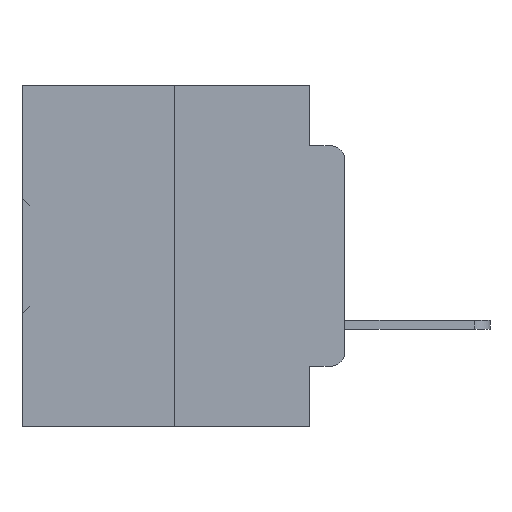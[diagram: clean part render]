
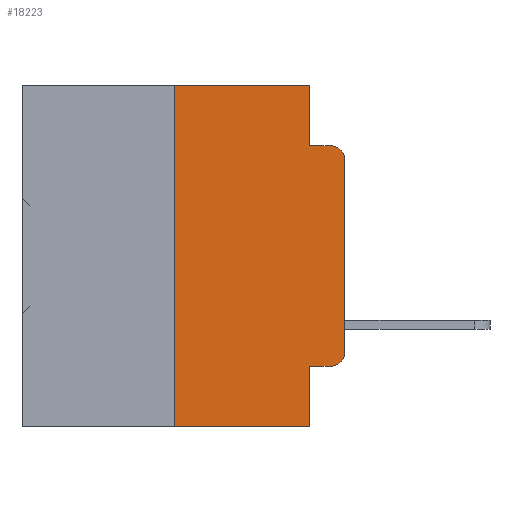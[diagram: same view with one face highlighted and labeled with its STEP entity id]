
A CAD part, left-side view. The second image highlights one B-rep face of the part: STEP entity #18223.
In plain terms, the highlighted planar face has unit normal (-1, 0, 0).
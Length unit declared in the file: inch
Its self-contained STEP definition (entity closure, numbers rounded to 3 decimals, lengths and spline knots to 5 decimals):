
#639 = VERTEX_POINT ( 'NONE', #9170 ) ;
#1669 = VECTOR ( 'NONE', #2910, 39.37008 ) ;
#1952 = CARTESIAN_POINT ( 'NONE',  ( 0., 0.25, 0. ) ) ;
#2910 = DIRECTION ( 'NONE',  ( 0., -1., 0. ) ) ;
#3035 = CARTESIAN_POINT ( 'NONE',  ( 0., 0.473, 0. ) ) ;
#3093 = DIRECTION ( 'NONE',  ( 0., 0., -1. ) ) ;
#4066 = CARTESIAN_POINT ( 'NONE',  ( 0., 0.02, -0.3915 ) ) ;
#5423 = DIRECTION ( 'NONE',  ( 0., -1., 0. ) ) ;
#5424 = VECTOR ( 'NONE', #35236, 39.37008 ) ;
#6036 = LINE ( 'NONE', #36632, #36297 ) ;
#6389 = DIRECTION ( 'NONE',  ( 1., 0., 0. ) ) ;
#6413 = EDGE_CURVE ( 'NONE', #38386, #11973, #16424, .T. ) ;
#7213 = VECTOR ( 'NONE', #23449, 39.37008 ) ;
#7255 = DIRECTION ( 'NONE',  ( 0., 0., -1. ) ) ;
#7344 = LINE ( 'NONE', #27933, #22648 ) ;
#7546 = DIRECTION ( 'NONE',  ( 0., -1., 0. ) ) ;
#7761 = VECTOR ( 'NONE', #5423, 39.37008 ) ;
#7992 = AXIS2_PLACEMENT_3D ( 'NONE', #4066, #25380, #7255 ) ;
#8568 = ORIENTED_EDGE ( 'NONE', *, *, #12694, .F. ) ;
#8886 = EDGE_LOOP ( 'NONE', ( #9324, #9096, #8568, #9856, #9718, #10100, #32846, #32036, #26861, #32527 ) ) ;
#9096 = ORIENTED_EDGE ( 'NONE', *, *, #18917, .T. ) ;
#9102 = VECTOR ( 'NONE', #36524, 39.37008 ) ;
#9170 = CARTESIAN_POINT ( 'NONE',  ( 0., 0.051, 0. ) ) ;
#9175 = VERTEX_POINT ( 'NONE', #12845 ) ;
#9254 = EDGE_CURVE ( 'NONE', #23897, #35153, #20009, .T. ) ;
#9324 = ORIENTED_EDGE ( 'NONE', *, *, #22839, .T. ) ;
#9718 = ORIENTED_EDGE ( 'NONE', *, *, #37402, .F. ) ;
#9856 = ORIENTED_EDGE ( 'NONE', *, *, #10630, .F. ) ;
#10017 = DIRECTION ( 'NONE',  ( -1., 0., 0. ) ) ;
#10100 = ORIENTED_EDGE ( 'NONE', *, *, #6413, .F. ) ;
#10434 = AXIS2_PLACEMENT_3D ( 'NONE', #3035, #6389, #27438 ) ;
#10630 = EDGE_CURVE ( 'NONE', #639, #30252, #28795, .T. ) ;
#11113 = LINE ( 'NONE', #24247, #1669 ) ;
#11973 = VERTEX_POINT ( 'NONE', #1952 ) ;
#12105 = CARTESIAN_POINT ( 'NONE',  ( 0., 0.473, -0.5 ) ) ;
#12694 = EDGE_CURVE ( 'NONE', #30252, #18925, #11113, .T. ) ;
#12845 = CARTESIAN_POINT ( 'NONE',  ( 0., 0.051, -0.5 ) ) ;
#14401 = CARTESIAN_POINT ( 'NONE',  ( 0., 0.25, 0. ) ) ;
#14724 = LINE ( 'NONE', #12105, #5424 ) ;
#14853 = CARTESIAN_POINT ( 'NONE',  ( 0., 0.473, 0. ) ) ;
#15561 = VERTEX_POINT ( 'NONE', #34172 ) ;
#15865 = CARTESIAN_POINT ( 'NONE',  ( 0., 0., -0.3915 ) ) ;
#16025 = LINE ( 'NONE', #14853, #7761 ) ;
#16424 = LINE ( 'NONE', #14401, #7213 ) ;
#18223 = ADVANCED_FACE ( 'NONE', ( #33778 ), #38359, .F. ) ;
#18917 = EDGE_CURVE ( 'NONE', #23589, #18925, #32056, .T. ) ;
#18925 = VERTEX_POINT ( 'NONE', #25049 ) ;
#19265 = AXIS2_PLACEMENT_3D ( 'NONE', #27866, #10017, #30638 ) ;
#19653 = EDGE_CURVE ( 'NONE', #15561, #23897, #6036, .T. ) ;
#20009 = CIRCLE ( 'NONE', #7992, 0.02 ) ;
#21164 = EDGE_CURVE ( 'NONE', #38386, #9175, #14724, .T. ) ;
#21243 = VECTOR ( 'NONE', #3093, 39.37008 ) ;
#22535 = CARTESIAN_POINT ( 'NONE',  ( 0., 0.25, -0.5 ) ) ;
#22648 = VECTOR ( 'NONE', #25120, 39.37008 ) ;
#22782 = CARTESIAN_POINT ( 'NONE',  ( 0., 0.051, -0.0885 ) ) ;
#22839 = EDGE_CURVE ( 'NONE', #35153, #23589, #7344, .T. ) ;
#23449 = DIRECTION ( 'NONE',  ( 0., 0., 1. ) ) ;
#23519 = CARTESIAN_POINT ( 'NONE',  ( 0., 0.02, -0.4115 ) ) ;
#23589 = VERTEX_POINT ( 'NONE', #33251 ) ;
#23897 = VERTEX_POINT ( 'NONE', #23519 ) ;
#24247 = CARTESIAN_POINT ( 'NONE',  ( 0., 0.051, -0.0885 ) ) ;
#25049 = CARTESIAN_POINT ( 'NONE',  ( 0., 0.02, -0.0885 ) ) ;
#25120 = DIRECTION ( 'NONE',  ( 0., 0., 1. ) ) ;
#25194 = LINE ( 'NONE', #25410, #9102 ) ;
#25380 = DIRECTION ( 'NONE',  ( -1., 0., 0. ) ) ;
#25410 = CARTESIAN_POINT ( 'NONE',  ( 0., 0.051, 0. ) ) ;
#26861 = ORIENTED_EDGE ( 'NONE', *, *, #19653, .T. ) ;
#27438 = DIRECTION ( 'NONE',  ( 0., 0., -1. ) ) ;
#27866 = CARTESIAN_POINT ( 'NONE',  ( 0., 0.02, -0.1085 ) ) ;
#27933 = CARTESIAN_POINT ( 'NONE',  ( 0., 0., 0. ) ) ;
#28795 = LINE ( 'NONE', #35549, #21243 ) ;
#30252 = VERTEX_POINT ( 'NONE', #22782 ) ;
#30638 = DIRECTION ( 'NONE',  ( 0., 0., -1. ) ) ;
#32036 = ORIENTED_EDGE ( 'NONE', *, *, #38380, .F. ) ;
#32056 = CIRCLE ( 'NONE', #19265, 0.02 ) ;
#32527 = ORIENTED_EDGE ( 'NONE', *, *, #9254, .T. ) ;
#32846 = ORIENTED_EDGE ( 'NONE', *, *, #21164, .T. ) ;
#33251 = CARTESIAN_POINT ( 'NONE',  ( 0., 0., -0.1085 ) ) ;
#33778 = FACE_OUTER_BOUND ( 'NONE', #8886, .T. ) ;
#34172 = CARTESIAN_POINT ( 'NONE',  ( 0., 0.051, -0.4115 ) ) ;
#35153 = VERTEX_POINT ( 'NONE', #15865 ) ;
#35236 = DIRECTION ( 'NONE',  ( 0., -1., 0. ) ) ;
#35549 = CARTESIAN_POINT ( 'NONE',  ( 0., 0.051, 0. ) ) ;
#36297 = VECTOR ( 'NONE', #7546, 39.37008 ) ;
#36524 = DIRECTION ( 'NONE',  ( 0., 0., -1. ) ) ;
#36632 = CARTESIAN_POINT ( 'NONE',  ( 0., 0.051, -0.4115 ) ) ;
#37402 = EDGE_CURVE ( 'NONE', #11973, #639, #16025, .T. ) ;
#38359 = PLANE ( 'NONE',  #10434 ) ;
#38380 = EDGE_CURVE ( 'NONE', #15561, #9175, #25194, .T. ) ;
#38386 = VERTEX_POINT ( 'NONE', #22535 ) ;
